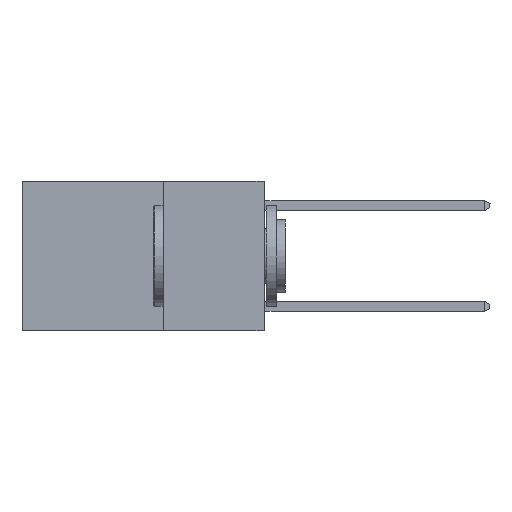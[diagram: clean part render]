
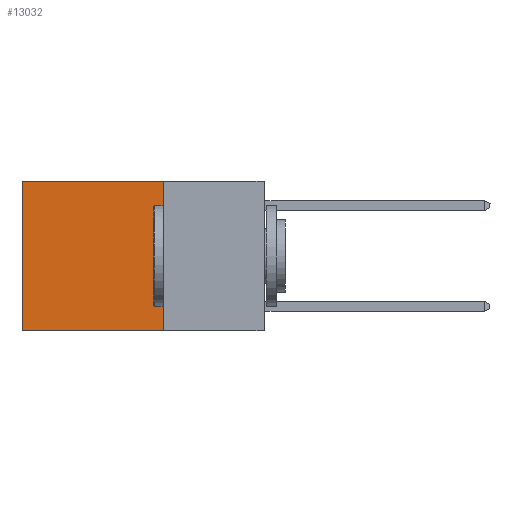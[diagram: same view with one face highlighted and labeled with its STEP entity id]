
A CAD part, left-side view. The second image highlights one B-rep face of the part: STEP entity #13032.
In plain terms, the highlighted planar face has unit normal (-1, 0, 0).
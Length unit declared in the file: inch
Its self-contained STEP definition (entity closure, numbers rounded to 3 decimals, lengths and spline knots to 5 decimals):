
#23 = CARTESIAN_POINT ( 'NONE',  ( 0.2625, 0.25, 0. ) ) ;
#51 = CARTESIAN_POINT ( 'NONE',  ( 0.2625, 0.25, -0.37 ) ) ;
#329 = CARTESIAN_POINT ( 'NONE',  ( 0.2625, 0.6, -0.37 ) ) ;
#492 = VERTEX_POINT ( 'NONE', #329 ) ;
#681 = LINE ( 'NONE', #17079, #19079 ) ;
#1070 = CARTESIAN_POINT ( 'NONE',  ( 0.2625, 0.25, -0.37 ) ) ;
#1699 = LINE ( 'NONE', #8812, #16063 ) ;
#1714 = FACE_OUTER_BOUND ( 'NONE', #7270, .T. ) ;
#1912 = DIRECTION ( 'NONE',  ( 1., 0., 0. ) ) ;
#2403 = EDGE_CURVE ( 'NONE', #2855, #492, #681, .T. ) ;
#2774 = ORIENTED_EDGE ( 'NONE', *, *, #3629, .F. ) ;
#2855 = VERTEX_POINT ( 'NONE', #6512 ) ;
#3270 = VECTOR ( 'NONE', #17880, 39.37008 ) ;
#3629 = EDGE_CURVE ( 'NONE', #5693, #492, #14878, .T. ) ;
#5193 = DIRECTION ( 'NONE',  ( 0., 0., -1. ) ) ;
#5693 = VERTEX_POINT ( 'NONE', #1070 ) ;
#6006 = EDGE_CURVE ( 'NONE', #16898, #5693, #6565, .T. ) ;
#6397 = ORIENTED_EDGE ( 'NONE', *, *, #9014, .T. ) ;
#6512 = CARTESIAN_POINT ( 'NONE',  ( 0.2625, 0.6, 0. ) ) ;
#6565 = LINE ( 'NONE', #11352, #14109 ) ;
#7270 = EDGE_LOOP ( 'NONE', ( #14653, #2774, #10512, #6397 ) ) ;
#8812 = CARTESIAN_POINT ( 'NONE',  ( 0.2625, 0.25, 0. ) ) ;
#8901 = AXIS2_PLACEMENT_3D ( 'NONE', #13826, #1912, #13730 ) ;
#9014 = EDGE_CURVE ( 'NONE', #16898, #2855, #1699, .T. ) ;
#9752 = DIRECTION ( 'NONE',  ( 0., 0., -1. ) ) ;
#10512 = ORIENTED_EDGE ( 'NONE', *, *, #6006, .F. ) ;
#11352 = CARTESIAN_POINT ( 'NONE',  ( 0.2625, 0.25, 0. ) ) ;
#13032 = ADVANCED_FACE ( 'NONE', ( #1714 ), #15196, .F. ) ;
#13730 = DIRECTION ( 'NONE',  ( 0., 0., -1. ) ) ;
#13826 = CARTESIAN_POINT ( 'NONE',  ( 0.2625, 0.25, 0. ) ) ;
#14109 = VECTOR ( 'NONE', #5193, 39.37008 ) ;
#14653 = ORIENTED_EDGE ( 'NONE', *, *, #2403, .T. ) ;
#14878 = LINE ( 'NONE', #51, #3270 ) ;
#14988 = DIRECTION ( 'NONE',  ( 0., 1., 0. ) ) ;
#15196 = PLANE ( 'NONE',  #8901 ) ;
#16063 = VECTOR ( 'NONE', #14988, 39.37008 ) ;
#16898 = VERTEX_POINT ( 'NONE', #23 ) ;
#17079 = CARTESIAN_POINT ( 'NONE',  ( 0.2625, 0.6, 0. ) ) ;
#17880 = DIRECTION ( 'NONE',  ( 0., 1., 0. ) ) ;
#19079 = VECTOR ( 'NONE', #9752, 39.37008 ) ;
